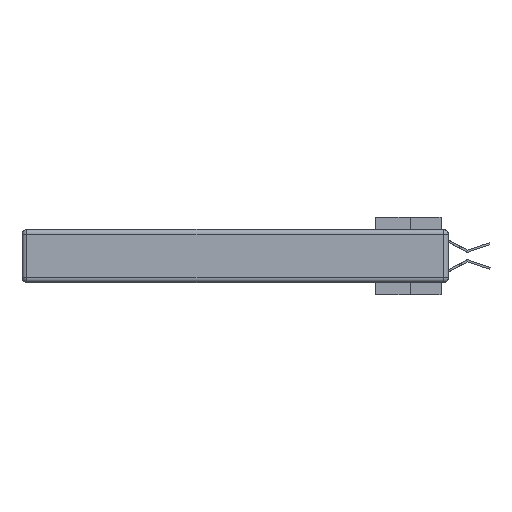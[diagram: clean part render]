
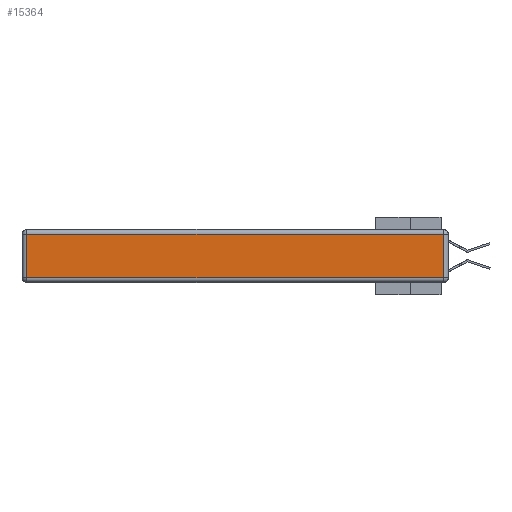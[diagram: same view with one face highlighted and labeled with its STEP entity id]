
A CAD part, left-side view. The second image highlights one B-rep face of the part: STEP entity #15364.
In plain terms, the highlighted planar face has unit normal (-1, 0, 0).
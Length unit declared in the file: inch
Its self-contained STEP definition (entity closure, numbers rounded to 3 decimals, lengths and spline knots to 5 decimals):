
#826 = LINE ( 'NONE', #24771, #1803 ) ;
#1080 = CARTESIAN_POINT ( 'NONE',  ( 0., 2.72, -0.03 ) ) ;
#1249 = DIRECTION ( 'NONE',  ( -1., 0., 0. ) ) ;
#1803 = VECTOR ( 'NONE', #19812, 39.37008 ) ;
#2922 = EDGE_CURVE ( 'NONE', #18994, #4583, #4050, .T. ) ;
#3223 = VERTEX_POINT ( 'NONE', #1080 ) ;
#4050 = LINE ( 'NONE', #4199, #4792 ) ;
#4199 = CARTESIAN_POINT ( 'NONE',  ( 0., 0., -0.313 ) ) ;
#4339 = CARTESIAN_POINT ( 'NONE',  ( 0., 0., -0.343 ) ) ;
#4583 = VERTEX_POINT ( 'NONE', #29065 ) ;
#4792 = VECTOR ( 'NONE', #21003, 39.37008 ) ;
#6313 = VERTEX_POINT ( 'NONE', #19302 ) ;
#6491 = EDGE_LOOP ( 'NONE', ( #12973, #27967, #26227, #21430 ) ) ;
#6552 = EDGE_CURVE ( 'NONE', #6313, #3223, #18619, .T. ) ;
#7133 = DIRECTION ( 'NONE',  ( 0., 0., 1. ) ) ;
#7596 = LINE ( 'NONE', #14298, #19546 ) ;
#12973 = ORIENTED_EDGE ( 'NONE', *, *, #2922, .T. ) ;
#13572 = EDGE_CURVE ( 'NONE', #3223, #18994, #826, .T. ) ;
#14298 = CARTESIAN_POINT ( 'NONE',  ( 0., 0.03, -0.343 ) ) ;
#15364 = ADVANCED_FACE ( 'NONE', ( #17871 ), #25621, .T. ) ;
#17871 = FACE_OUTER_BOUND ( 'NONE', #6491, .T. ) ;
#18619 = LINE ( 'NONE', #28092, #23474 ) ;
#18994 = VERTEX_POINT ( 'NONE', #27012 ) ;
#19302 = CARTESIAN_POINT ( 'NONE',  ( 0., 0.03, -0.03 ) ) ;
#19546 = VECTOR ( 'NONE', #7133, 39.37008 ) ;
#19812 = DIRECTION ( 'NONE',  ( 0., 0., -1. ) ) ;
#20386 = DIRECTION ( 'NONE',  ( 0., 0., 1. ) ) ;
#21003 = DIRECTION ( 'NONE',  ( 0., -1., 0. ) ) ;
#21274 = AXIS2_PLACEMENT_3D ( 'NONE', #4339, #1249, #20386 ) ;
#21430 = ORIENTED_EDGE ( 'NONE', *, *, #13572, .T. ) ;
#23474 = VECTOR ( 'NONE', #23616, 39.37008 ) ;
#23616 = DIRECTION ( 'NONE',  ( 0., 1., 0. ) ) ;
#24771 = CARTESIAN_POINT ( 'NONE',  ( 0., 2.72, -0.343 ) ) ;
#25621 = PLANE ( 'NONE',  #21274 ) ;
#26227 = ORIENTED_EDGE ( 'NONE', *, *, #6552, .T. ) ;
#27012 = CARTESIAN_POINT ( 'NONE',  ( 0., 2.72, -0.313 ) ) ;
#27721 = EDGE_CURVE ( 'NONE', #4583, #6313, #7596, .T. ) ;
#27967 = ORIENTED_EDGE ( 'NONE', *, *, #27721, .T. ) ;
#28092 = CARTESIAN_POINT ( 'NONE',  ( 0., 2.75, -0.03 ) ) ;
#29065 = CARTESIAN_POINT ( 'NONE',  ( 0., 0.03, -0.313 ) ) ;
